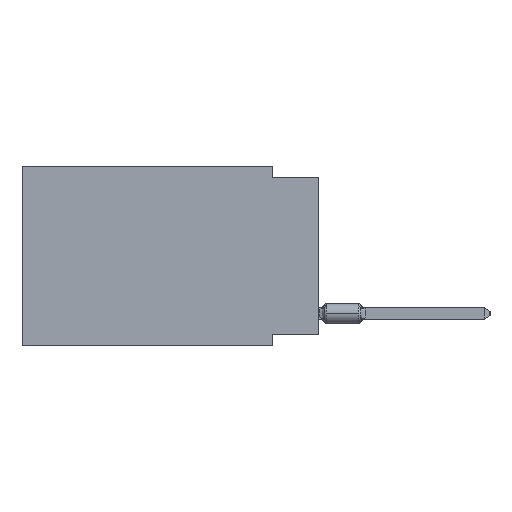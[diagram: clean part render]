
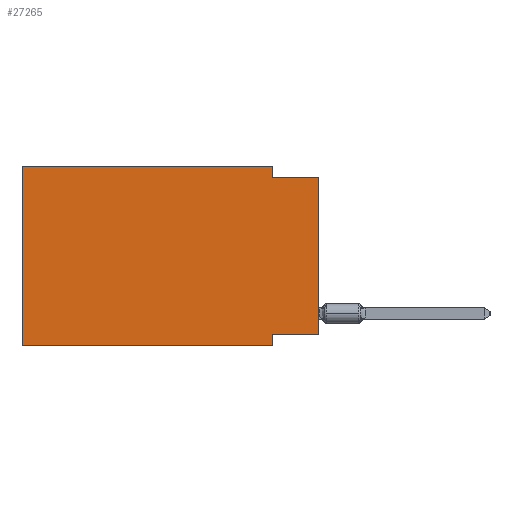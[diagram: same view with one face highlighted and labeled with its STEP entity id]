
A CAD part, left-side view. The second image highlights one B-rep face of the part: STEP entity #27265.
In plain terms, the highlighted planar face has unit normal (-1, 0, 0).
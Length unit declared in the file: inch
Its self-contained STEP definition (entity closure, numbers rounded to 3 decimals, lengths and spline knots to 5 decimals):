
#576 = AXIS2_PLACEMENT_3D ( 'NONE', #19504, #22999, #23215 ) ;
#1394 = CARTESIAN_POINT ( 'NONE',  ( 0., 0.645, -0.39 ) ) ;
#1670 = CARTESIAN_POINT ( 'NONE',  ( 0., 0., -0.025 ) ) ;
#2448 = CARTESIAN_POINT ( 'NONE',  ( 0., 0.1, -0.365 ) ) ;
#3042 = CARTESIAN_POINT ( 'NONE',  ( 0., 0.1, -0.39 ) ) ;
#3603 = ORIENTED_EDGE ( 'NONE', *, *, #14056, .F. ) ;
#3683 = PLANE ( 'NONE',  #576 ) ;
#5432 = CARTESIAN_POINT ( 'NONE',  ( 0., 0., -0.365 ) ) ;
#6096 = VECTOR ( 'NONE', #33865, 39.37008 ) ;
#6259 = VECTOR ( 'NONE', #31928, 39.37008 ) ;
#6300 = EDGE_CURVE ( 'NONE', #29477, #27274, #14622, .T. ) ;
#8046 = EDGE_CURVE ( 'NONE', #29477, #41678, #38453, .T. ) ;
#8074 = CARTESIAN_POINT ( 'NONE',  ( 0., 0.645, -0.39 ) ) ;
#8118 = DIRECTION ( 'NONE',  ( 0., -1., 0. ) ) ;
#9375 = DIRECTION ( 'NONE',  ( 0., 0., 1. ) ) ;
#9593 = LINE ( 'NONE', #23478, #17007 ) ;
#10023 = ORIENTED_EDGE ( 'NONE', *, *, #22365, .F. ) ;
#10110 = VECTOR ( 'NONE', #41874, 39.37008 ) ;
#10693 = VERTEX_POINT ( 'NONE', #33508 ) ;
#11878 = ORIENTED_EDGE ( 'NONE', *, *, #24709, .F. ) ;
#11972 = VERTEX_POINT ( 'NONE', #13970 ) ;
#12326 = ORIENTED_EDGE ( 'NONE', *, *, #37752, .F. ) ;
#12512 = CARTESIAN_POINT ( 'NONE',  ( 0., 0.1, 0. ) ) ;
#13970 = CARTESIAN_POINT ( 'NONE',  ( 0., 0.1, -0.025 ) ) ;
#14056 = EDGE_CURVE ( 'NONE', #41678, #38751, #24638, .T. ) ;
#14622 = LINE ( 'NONE', #1394, #34536 ) ;
#15227 = ORIENTED_EDGE ( 'NONE', *, *, #22101, .T. ) ;
#15637 = ORIENTED_EDGE ( 'NONE', *, *, #8046, .F. ) ;
#17007 = VECTOR ( 'NONE', #9375, 39.37008 ) ;
#17248 = VECTOR ( 'NONE', #37488, 39.37008 ) ;
#17592 = ORIENTED_EDGE ( 'NONE', *, *, #26326, .F. ) ;
#17901 = DIRECTION ( 'NONE',  ( 0., -1., 0. ) ) ;
#19504 = CARTESIAN_POINT ( 'NONE',  ( 0., 0.645, 0. ) ) ;
#20145 = FACE_OUTER_BOUND ( 'NONE', #30111, .T. ) ;
#20303 = LINE ( 'NONE', #36596, #34183 ) ;
#22101 = EDGE_CURVE ( 'NONE', #10693, #31581, #9593, .T. ) ;
#22365 = EDGE_CURVE ( 'NONE', #10693, #26750, #27990, .T. ) ;
#22999 = DIRECTION ( 'NONE',  ( 1., 0., 0. ) ) ;
#23215 = DIRECTION ( 'NONE',  ( 0., 0., -1. ) ) ;
#23478 = CARTESIAN_POINT ( 'NONE',  ( 0., 0., 0. ) ) ;
#24043 = CARTESIAN_POINT ( 'NONE',  ( 0., 0.645, 0. ) ) ;
#24638 = LINE ( 'NONE', #37873, #36749 ) ;
#24709 = EDGE_CURVE ( 'NONE', #11972, #31581, #40380, .T. ) ;
#25213 = CARTESIAN_POINT ( 'NONE',  ( 0., 0.645, 0. ) ) ;
#26326 = EDGE_CURVE ( 'NONE', #26750, #27274, #40334, .T. ) ;
#26750 = VERTEX_POINT ( 'NONE', #2448 ) ;
#27265 = ADVANCED_FACE ( 'NONE', ( #20145 ), #3683, .F. ) ;
#27274 = VERTEX_POINT ( 'NONE', #3042 ) ;
#27990 = LINE ( 'NONE', #5432, #10110 ) ;
#29477 = VERTEX_POINT ( 'NONE', #8074 ) ;
#29662 = DIRECTION ( 'NONE',  ( 0., 0., -1. ) ) ;
#30111 = EDGE_LOOP ( 'NONE', ( #15227, #11878, #12326, #3603, #15637, #42902, #17592, #10023 ) ) ;
#31581 = VERTEX_POINT ( 'NONE', #1670 ) ;
#31928 = DIRECTION ( 'NONE',  ( 0., 0., 1. ) ) ;
#33508 = CARTESIAN_POINT ( 'NONE',  ( 0., 0., -0.365 ) ) ;
#33865 = DIRECTION ( 'NONE',  ( 0., -1., 0. ) ) ;
#34183 = VECTOR ( 'NONE', #29662, 39.37008 ) ;
#34536 = VECTOR ( 'NONE', #8118, 39.37008 ) ;
#36596 = CARTESIAN_POINT ( 'NONE',  ( 0., 0.1, 0. ) ) ;
#36749 = VECTOR ( 'NONE', #17901, 39.37008 ) ;
#37117 = CARTESIAN_POINT ( 'NONE',  ( 0., 0., -0.025 ) ) ;
#37280 = CARTESIAN_POINT ( 'NONE',  ( 0., 0.1, -0.39 ) ) ;
#37488 = DIRECTION ( 'NONE',  ( 0., 0., -1. ) ) ;
#37752 = EDGE_CURVE ( 'NONE', #38751, #11972, #20303, .T. ) ;
#37873 = CARTESIAN_POINT ( 'NONE',  ( 0., 0.645, 0. ) ) ;
#38453 = LINE ( 'NONE', #25213, #6259 ) ;
#38751 = VERTEX_POINT ( 'NONE', #12512 ) ;
#40334 = LINE ( 'NONE', #37280, #17248 ) ;
#40380 = LINE ( 'NONE', #37117, #6096 ) ;
#41678 = VERTEX_POINT ( 'NONE', #24043 ) ;
#41874 = DIRECTION ( 'NONE',  ( 0., 1., 0. ) ) ;
#42902 = ORIENTED_EDGE ( 'NONE', *, *, #6300, .T. ) ;
